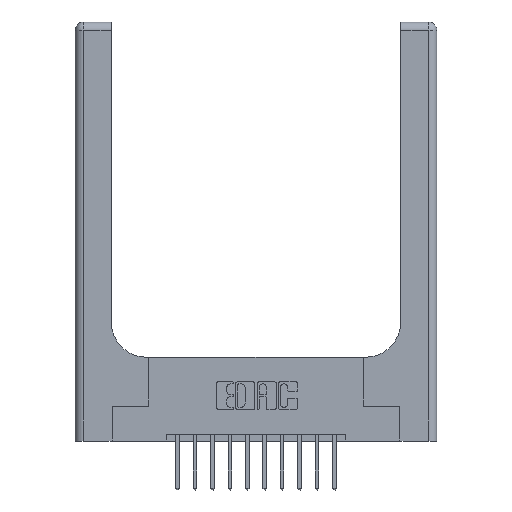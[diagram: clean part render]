
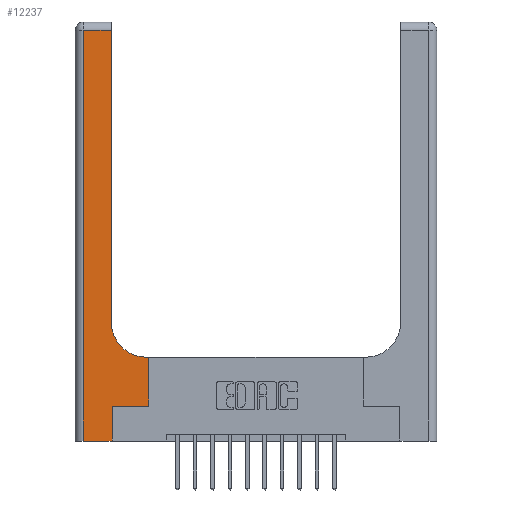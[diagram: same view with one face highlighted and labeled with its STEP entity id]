
A CAD part, top view. The second image highlights one B-rep face of the part: STEP entity #12237.
In plain terms, the highlighted planar face has unit normal (0, 0, 1).
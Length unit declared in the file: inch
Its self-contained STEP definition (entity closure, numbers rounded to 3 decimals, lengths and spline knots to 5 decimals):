
#10 = VERTEX_POINT ( 'NONE', #11172 ) ;
#258 = ORIENTED_EDGE ( 'NONE', *, *, #7091, .T. ) ;
#886 = VERTEX_POINT ( 'NONE', #2285 ) ;
#1134 = VERTEX_POINT ( 'NONE', #10565 ) ;
#1544 = VECTOR ( 'NONE', #14609, 39.37008 ) ;
#1549 = VERTEX_POINT ( 'NONE', #12598 ) ;
#2047 = EDGE_CURVE ( 'NONE', #886, #8717, #14083, .T. ) ;
#2285 = CARTESIAN_POINT ( 'NONE',  ( 0.06, 0., 0.37 ) ) ;
#2494 = CARTESIAN_POINT ( 'NONE',  ( 0.265, 0., 0.37 ) ) ;
#2518 = EDGE_CURVE ( 'NONE', #8717, #15526, #15839, .T. ) ;
#2538 = ORIENTED_EDGE ( 'NONE', *, *, #8665, .T. ) ;
#2590 = FACE_OUTER_BOUND ( 'NONE', #7283, .T. ) ;
#2739 = CARTESIAN_POINT ( 'NONE',  ( 0., 0., 0.37 ) ) ;
#3429 = LINE ( 'NONE', #8688, #14639 ) ;
#3695 = CARTESIAN_POINT ( 'NONE',  ( 0.51, 0.6, 0.37 ) ) ;
#4101 = LINE ( 'NONE', #5103, #11068 ) ;
#4336 = ORIENTED_EDGE ( 'NONE', *, *, #9837, .T. ) ;
#4562 = DIRECTION ( 'NONE',  ( 0., 0., -1. ) ) ;
#4831 = ORIENTED_EDGE ( 'NONE', *, *, #5236, .T. ) ;
#4925 = LINE ( 'NONE', #13339, #8597 ) ;
#5049 = DIRECTION ( 'NONE',  ( 0., 0., -1. ) ) ;
#5103 = CARTESIAN_POINT ( 'NONE',  ( 0.528, 0.25, 0.37 ) ) ;
#5236 = EDGE_CURVE ( 'NONE', #15212, #11070, #7763, .T. ) ;
#5908 = ORIENTED_EDGE ( 'NONE', *, *, #2518, .T. ) ;
#5960 = VECTOR ( 'NONE', #8089, 39.37008 ) ;
#5981 = DIRECTION ( 'NONE',  ( 0., 1., 0. ) ) ;
#6333 = LINE ( 'NONE', #9371, #5960 ) ;
#6573 = VECTOR ( 'NONE', #12603, 39.37008 ) ;
#6799 = AXIS2_PLACEMENT_3D ( 'NONE', #15027, #5049, #7647 ) ;
#7091 = EDGE_CURVE ( 'NONE', #11070, #1134, #10627, .T. ) ;
#7102 = CARTESIAN_POINT ( 'NONE',  ( 0.26, 0.6, 0.37 ) ) ;
#7184 = ORIENTED_EDGE ( 'NONE', *, *, #2047, .T. ) ;
#7283 = EDGE_LOOP ( 'NONE', ( #13595, #2538, #10065, #7184, #5908, #15189, #4336, #4831, #258 ) ) ;
#7647 = DIRECTION ( 'NONE',  ( 1., 0., 0. ) ) ;
#7763 = LINE ( 'NONE', #7102, #10461 ) ;
#7796 = CARTESIAN_POINT ( 'NONE',  ( 0.265, 0.25, 0.37 ) ) ;
#8089 = DIRECTION ( 'NONE',  ( 0., -1., 0. ) ) ;
#8384 = DIRECTION ( 'NONE',  ( -1., 0., 0. ) ) ;
#8597 = VECTOR ( 'NONE', #5981, 39.37008 ) ;
#8665 = EDGE_CURVE ( 'NONE', #11656, #1549, #3429, .T. ) ;
#8688 = CARTESIAN_POINT ( 'NONE',  ( 0., 2.94, 0.37 ) ) ;
#8717 = VERTEX_POINT ( 'NONE', #2494 ) ;
#8895 = EDGE_CURVE ( 'NONE', #1549, #886, #6333, .T. ) ;
#9281 = DIRECTION ( 'NONE',  ( 0., 1., 0. ) ) ;
#9337 = LINE ( 'NONE', #11000, #1544 ) ;
#9371 = CARTESIAN_POINT ( 'NONE',  ( 0.06, 3., 0.37 ) ) ;
#9837 = EDGE_CURVE ( 'NONE', #10, #15212, #4101, .T. ) ;
#10065 = ORIENTED_EDGE ( 'NONE', *, *, #8895, .T. ) ;
#10461 = VECTOR ( 'NONE', #10935, 39.37008 ) ;
#10565 = CARTESIAN_POINT ( 'NONE',  ( 0.26, 0.85, 0.37 ) ) ;
#10627 = CIRCLE ( 'NONE', #6799, 0.25 ) ;
#10725 = PLANE ( 'NONE',  #15737 ) ;
#10935 = DIRECTION ( 'NONE',  ( -1., 0., 0. ) ) ;
#11000 = CARTESIAN_POINT ( 'NONE',  ( 0.265, 0.25, 0.37 ) ) ;
#11006 = CARTESIAN_POINT ( 'NONE',  ( 0.528, 0.6, 0.37 ) ) ;
#11068 = VECTOR ( 'NONE', #13742, 39.37008 ) ;
#11070 = VERTEX_POINT ( 'NONE', #3695 ) ;
#11172 = CARTESIAN_POINT ( 'NONE',  ( 0.528, 0.25, 0.37 ) ) ;
#11278 = DIRECTION ( 'NONE',  ( -1., 0., 0. ) ) ;
#11656 = VERTEX_POINT ( 'NONE', #12343 ) ;
#12237 = ADVANCED_FACE ( 'NONE', ( #2590 ), #10725, .F. ) ;
#12343 = CARTESIAN_POINT ( 'NONE',  ( 0.26, 2.94, 0.37 ) ) ;
#12543 = VECTOR ( 'NONE', #9281, 39.37008 ) ;
#12598 = CARTESIAN_POINT ( 'NONE',  ( 0.06, 2.94, 0.37 ) ) ;
#12603 = DIRECTION ( 'NONE',  ( 1., 0., 0. ) ) ;
#12966 = EDGE_CURVE ( 'NONE', #1134, #11656, #4925, .T. ) ;
#13339 = CARTESIAN_POINT ( 'NONE',  ( 0.26, 3., 0.37 ) ) ;
#13595 = ORIENTED_EDGE ( 'NONE', *, *, #12966, .T. ) ;
#13742 = DIRECTION ( 'NONE',  ( 0., 1., 0. ) ) ;
#14053 = EDGE_CURVE ( 'NONE', #15526, #10, #9337, .T. ) ;
#14083 = LINE ( 'NONE', #2739, #6573 ) ;
#14195 = CARTESIAN_POINT ( 'NONE',  ( 0.265, 0., 0.37 ) ) ;
#14609 = DIRECTION ( 'NONE',  ( 1., 0., 0. ) ) ;
#14639 = VECTOR ( 'NONE', #11278, 39.37008 ) ;
#15027 = CARTESIAN_POINT ( 'NONE',  ( 0.51, 0.85, 0.37 ) ) ;
#15189 = ORIENTED_EDGE ( 'NONE', *, *, #14053, .T. ) ;
#15212 = VERTEX_POINT ( 'NONE', #11006 ) ;
#15526 = VERTEX_POINT ( 'NONE', #7796 ) ;
#15737 = AXIS2_PLACEMENT_3D ( 'NONE', #15789, #4562, #8384 ) ;
#15789 = CARTESIAN_POINT ( 'NONE',  ( 0., 3., 0.37 ) ) ;
#15839 = LINE ( 'NONE', #14195, #12543 ) ;
